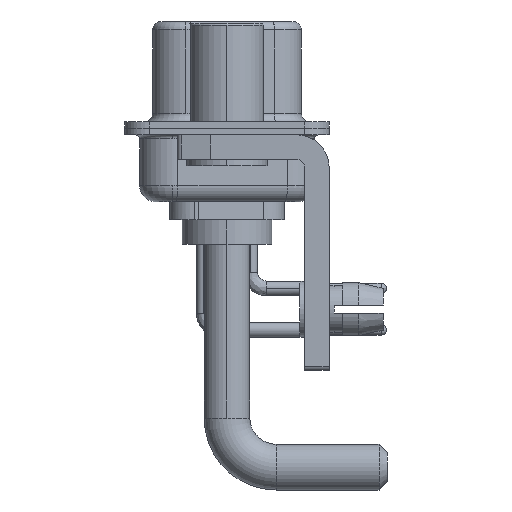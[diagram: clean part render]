
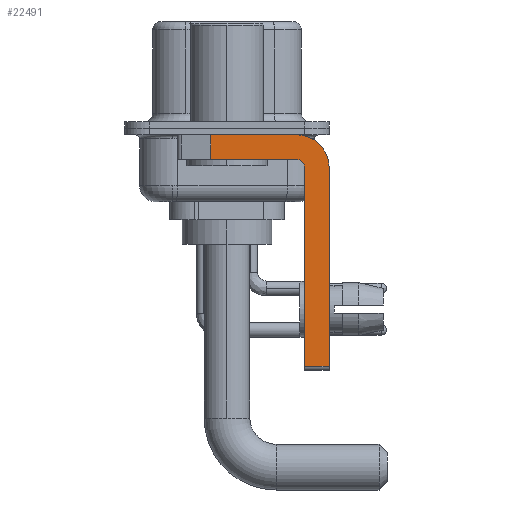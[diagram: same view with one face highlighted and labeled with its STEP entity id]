
A CAD part, left-side view. The second image highlights one B-rep face of the part: STEP entity #22491.
In plain terms, the highlighted planar face has unit normal (-1, 0, 0).
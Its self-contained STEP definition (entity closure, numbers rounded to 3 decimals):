
#17 = CARTESIAN_POINT ( 'NONE',  ( -2.9, -4.25, -1.9 ) ) ;
#1742 = PLANE ( 'NONE',  #27162 ) ;
#2125 = EDGE_CURVE ( 'NONE', #14986, #29067, #17902, .T. ) ;
#2981 = EDGE_CURVE ( 'NONE', #20091, #32247, #19327, .T. ) ;
#3259 = CIRCLE ( 'NONE', #31762, 2. ) ;
#3264 = LINE ( 'NONE', #10379, #12218 ) ;
#3729 = FACE_OUTER_BOUND ( 'NONE', #22142, .T. ) ;
#3834 = CARTESIAN_POINT ( 'NONE',  ( -2.9, -4.25, -1.9 ) ) ;
#4114 = LINE ( 'NONE', #23964, #21582 ) ;
#4290 = CIRCLE ( 'NONE', #13272, 0.5 ) ;
#4446 = CARTESIAN_POINT ( 'NONE',  ( -2.9, 0.978, -0.4 ) ) ;
#5224 = VERTEX_POINT ( 'NONE', #14249 ) ;
#5225 = VECTOR ( 'NONE', #8557, 1000. ) ;
#5608 = VECTOR ( 'NONE', #27625, 1000. ) ;
#6746 = DIRECTION ( 'NONE',  ( 0., 0., 1. ) ) ;
#7024 = CARTESIAN_POINT ( 'NONE',  ( -2.9, -4.25, -2.4 ) ) ;
#7390 = EDGE_CURVE ( 'NONE', #32247, #14986, #4290, .T. ) ;
#7531 = CARTESIAN_POINT ( 'NONE',  ( -2.9, -6.25, -14.55 ) ) ;
#7768 = ORIENTED_EDGE ( 'NONE', *, *, #7390, .F. ) ;
#8557 = DIRECTION ( 'NONE',  ( 0., -1., 0. ) ) ;
#8968 = ORIENTED_EDGE ( 'NONE', *, *, #2125, .F. ) ;
#9994 = DIRECTION ( 'NONE',  ( -1., 0., 0. ) ) ;
#10379 = CARTESIAN_POINT ( 'NONE',  ( -2.9, -6.25, -2.4 ) ) ;
#10703 = VERTEX_POINT ( 'NONE', #4446 ) ;
#10780 = CARTESIAN_POINT ( 'NONE',  ( -2.9, 0.978, -1.9 ) ) ;
#10921 = CARTESIAN_POINT ( 'NONE',  ( -2.9, -4.75, -14.55 ) ) ;
#11406 = DIRECTION ( 'NONE',  ( 0., -1., 0. ) ) ;
#12218 = VECTOR ( 'NONE', #28704, 1000. ) ;
#13272 = AXIS2_PLACEMENT_3D ( 'NONE', #7024, #9994, #17281 ) ;
#13682 = CARTESIAN_POINT ( 'NONE',  ( -2.9, 3., -0.4 ) ) ;
#13820 = ORIENTED_EDGE ( 'NONE', *, *, #17682, .F. ) ;
#13993 = CARTESIAN_POINT ( 'NONE',  ( -2.9, -4.25, -2.4 ) ) ;
#14249 = CARTESIAN_POINT ( 'NONE',  ( -2.9, -4.25, -0.4 ) ) ;
#14371 = ORIENTED_EDGE ( 'NONE', *, *, #17225, .F. ) ;
#14376 = VERTEX_POINT ( 'NONE', #7531 ) ;
#14986 = VERTEX_POINT ( 'NONE', #3834 ) ;
#15181 = LINE ( 'NONE', #13682, #5225 ) ;
#15225 = ORIENTED_EDGE ( 'NONE', *, *, #26411, .F. ) ;
#15349 = CARTESIAN_POINT ( 'NONE',  ( -2.9, -6.25, -2.4 ) ) ;
#15972 = DIRECTION ( 'NONE',  ( 1., 0., 0. ) ) ;
#16866 = ORIENTED_EDGE ( 'NONE', *, *, #2981, .F. ) ;
#17225 = EDGE_CURVE ( 'NONE', #26305, #14376, #3264, .T. ) ;
#17281 = DIRECTION ( 'NONE',  ( 0., 0., 1. ) ) ;
#17682 = EDGE_CURVE ( 'NONE', #5224, #26305, #3259, .T. ) ;
#17902 = LINE ( 'NONE', #17, #5608 ) ;
#18958 = DIRECTION ( 'NONE',  ( 0., 0., -1. ) ) ;
#19327 = LINE ( 'NONE', #31364, #32050 ) ;
#20091 = VERTEX_POINT ( 'NONE', #10921 ) ;
#20533 = CARTESIAN_POINT ( 'NONE',  ( -2.9, 0.978, -1.9 ) ) ;
#20876 = DIRECTION ( 'NONE',  ( 0., 0., -1. ) ) ;
#21582 = VECTOR ( 'NONE', #11406, 1000. ) ;
#22142 = EDGE_LOOP ( 'NONE', ( #15225, #24740, #8968, #7768, #16866, #24577, #14371, #13820 ) ) ;
#22491 = ADVANCED_FACE ( 'NONE', ( #3729 ), #1742, .F. ) ;
#23063 = DIRECTION ( 'NONE',  ( 0., 0., -1. ) ) ;
#23340 = LINE ( 'NONE', #10780, #26762 ) ;
#23964 = CARTESIAN_POINT ( 'NONE',  ( -2.9, -4.25, -14.55 ) ) ;
#24577 = ORIENTED_EDGE ( 'NONE', *, *, #26206, .T. ) ;
#24611 = EDGE_CURVE ( 'NONE', #10703, #29067, #23340, .T. ) ;
#24740 = ORIENTED_EDGE ( 'NONE', *, *, #24611, .T. ) ;
#26206 = EDGE_CURVE ( 'NONE', #20091, #14376, #4114, .T. ) ;
#26305 = VERTEX_POINT ( 'NONE', #15349 ) ;
#26411 = EDGE_CURVE ( 'NONE', #10703, #5224, #15181, .T. ) ;
#26762 = VECTOR ( 'NONE', #20876, 1000. ) ;
#27162 = AXIS2_PLACEMENT_3D ( 'NONE', #13993, #31823, #18958 ) ;
#27625 = DIRECTION ( 'NONE',  ( 0., 1., 0. ) ) ;
#28704 = DIRECTION ( 'NONE',  ( 0., 0., -1. ) ) ;
#29067 = VERTEX_POINT ( 'NONE', #20533 ) ;
#29718 = CARTESIAN_POINT ( 'NONE',  ( -2.9, -4.75, -2.4 ) ) ;
#30647 = CARTESIAN_POINT ( 'NONE',  ( -2.9, -4.25, -2.4 ) ) ;
#31364 = CARTESIAN_POINT ( 'NONE',  ( -2.9, -4.75, -14.8 ) ) ;
#31762 = AXIS2_PLACEMENT_3D ( 'NONE', #30647, #15972, #23063 ) ;
#31823 = DIRECTION ( 'NONE',  ( 1., 0., 0. ) ) ;
#32050 = VECTOR ( 'NONE', #6746, 1000. ) ;
#32247 = VERTEX_POINT ( 'NONE', #29718 ) ;
